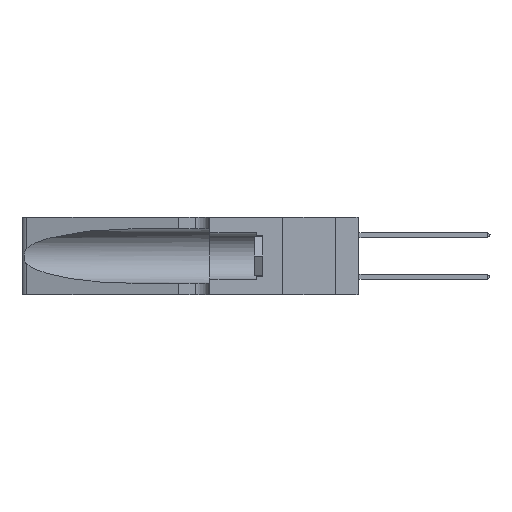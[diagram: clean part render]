
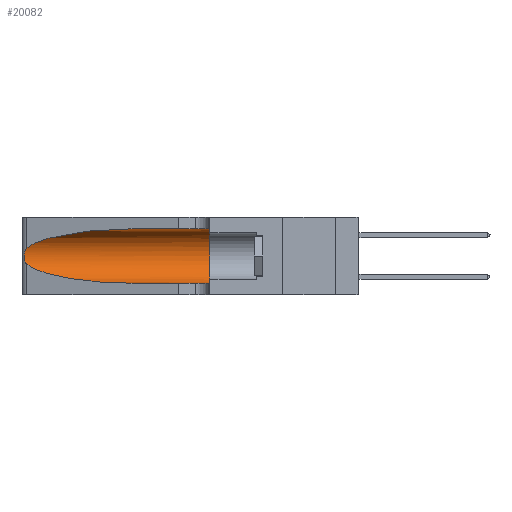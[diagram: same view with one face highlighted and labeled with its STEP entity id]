
A CAD part, left-side view. The second image highlights one B-rep face of the part: STEP entity #20082.
In plain terms, the highlighted cylindrical face has radius 3.308 mm (diameter 6.617 mm), a partial arc.
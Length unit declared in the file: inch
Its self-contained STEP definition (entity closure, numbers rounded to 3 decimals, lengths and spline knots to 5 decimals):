
#1 = VECTOR ( 'NONE', #4789, 39.37008 ) ;
#496 = VERTEX_POINT ( 'NONE', #16789 ) ;
#528 = ORIENTED_EDGE ( 'NONE', *, *, #17644, .T. ) ;
#596 = CARTESIAN_POINT ( 'NONE',  ( 0.26017, 1.23833, 0.17102 ) ) ;
#1968 = VECTOR ( 'NONE', #13540, 39.37008 ) ;
#2233 = VERTEX_POINT ( 'NONE', #7448 ) ;
#2292 = CARTESIAN_POINT ( 'NONE',  ( 0.1305, 1.61858, 0.31525 ) ) ;
#2737 = LINE ( 'NONE', #11096, #1968 ) ;
#2956 = CARTESIAN_POINT ( 'NONE',  ( 0.25555, 1.22994, 0.2215 ) ) ;
#3065 = CARTESIAN_POINT ( 'NONE',  ( 0.25789, 1.23486, 0.15765 ) ) ;
#3629 = EDGE_CURVE ( 'NONE', #496, #17994, #12127, .T. ) ;
#4636 = EDGE_CURVE ( 'NONE', #2233, #13091, #5561, .T. ) ;
#4789 = DIRECTION ( 'NONE',  ( 0., -1., 0. ) ) ;
#5550 = CARTESIAN_POINT ( 'NONE',  ( 0.25555, 1.22993, 0.14849 ) ) ;
#5561 = CIRCLE ( 'NONE', #5990, 0.13025 ) ;
#5990 = AXIS2_PLACEMENT_3D ( 'NONE', #22006, #7514, #24447 ) ;
#6458 =( BOUNDED_CURVE ( )  B_SPLINE_CURVE ( 3, ( #21441, #11854, #28164, #13734 ),
 .UNSPECIFIED., .F., .F. ) 
 B_SPLINE_CURVE_WITH_KNOTS ( ( 4, 4 ),
 ( 3.44316, 4.71239 ),
 .UNSPECIFIED. ) 
 CURVE ( )  GEOMETRIC_REPRESENTATION_ITEM ( )  RATIONAL_B_SPLINE_CURVE ( ( 1., 0.87, 0.87, 1. ) ) 
 REPRESENTATION_ITEM ( '' )  );
#7448 = CARTESIAN_POINT ( 'NONE',  ( 0.1305, 0.35, 0.31525 ) ) ;
#7514 = DIRECTION ( 'NONE',  ( 0., 1., 0. ) ) ;
#8742 = EDGE_CURVE ( 'NONE', #17994, #12324, #6458, .T. ) ;
#9635 = CARTESIAN_POINT ( 'NONE',  ( 0.2373, 1.15595, 0.28018 ) ) ;
#10351 = CARTESIAN_POINT ( 'NONE',  ( 0.25787, 1.23484, 0.2124 ) ) ;
#10816 = CARTESIAN_POINT ( 'NONE',  ( 0.25487, 1.22718, 0.14631 ) ) ;
#11096 = CARTESIAN_POINT ( 'NONE',  ( 0.1305, 1.61858, 0.05475 ) ) ;
#11854 = CARTESIAN_POINT ( 'NONE',  ( 0.2373, 1.15595, 0.08982 ) ) ;
#11987 = CARTESIAN_POINT ( 'NONE',  ( 0.18966, 0.96281, 0.31525 ) ) ;
#12127 = B_SPLINE_CURVE_WITH_KNOTS ( 'NONE', 3,
 ( #29557, #2956, #24833, #10351, #27231, #12792, #29659, #15218, #596, #17648, #3065, #20070, #5550, #22483 ),
 .UNSPECIFIED., .F., .F.,
 ( 4, 2, 2, 2, 2, 2, 4 ),
 ( 0., 0.00027, 0.00053, 0.00107, 0.0016, 0.00187, 0.00214 ),
 .UNSPECIFIED. ) ;
#12265 = VERTEX_POINT ( 'NONE', #16935 ) ;
#12316 = CARTESIAN_POINT ( 'NONE',  ( 0.1305, 0.72297, 0.05475 ) ) ;
#12324 = VERTEX_POINT ( 'NONE', #12316 ) ;
#12792 = CARTESIAN_POINT ( 'NONE',  ( 0.26018, 1.23835, 0.19895 ) ) ;
#13091 = VERTEX_POINT ( 'NONE', #19764 ) ;
#13110 = CYLINDRICAL_SURFACE ( 'NONE', #20943, 0.13025 ) ;
#13540 = DIRECTION ( 'NONE',  ( 0., -1., 0. ) ) ;
#13734 = CARTESIAN_POINT ( 'NONE',  ( 0.1305, 0.72297, 0.05475 ) ) ;
#14319 = CARTESIAN_POINT ( 'NONE',  ( 0.1305, 0.72297, 0.31525 ) ) ;
#14555 = DIRECTION ( 'NONE',  ( 0., 0., -1. ) ) ;
#14659 = ORIENTED_EDGE ( 'NONE', *, *, #3629, .T. ) ;
#15218 = CARTESIAN_POINT ( 'NONE',  ( 0.26075, 1.23896, 0.178 ) ) ;
#15238 = EDGE_LOOP ( 'NONE', ( #528, #14659, #27485, #29419, #21823, #20385 ) ) ;
#16789 = CARTESIAN_POINT ( 'NONE',  ( 0.25487, 1.22718, 0.22369 ) ) ;
#16935 = CARTESIAN_POINT ( 'NONE',  ( 0.1305, 0.72297, 0.31525 ) ) ;
#16963 = DIRECTION ( 'NONE',  ( 0., -1., 0. ) ) ;
#17644 = EDGE_CURVE ( 'NONE', #12265, #496, #21013, .T. ) ;
#17648 = CARTESIAN_POINT ( 'NONE',  ( 0.25856, 1.23593, 0.16098 ) ) ;
#17994 = VERTEX_POINT ( 'NONE', #10816 ) ;
#19459 = LINE ( 'NONE', #2292, #1 ) ;
#19764 = CARTESIAN_POINT ( 'NONE',  ( 0.1305, 0.35, 0.05475 ) ) ;
#20070 = CARTESIAN_POINT ( 'NONE',  ( 0.25639, 1.23186, 0.15144 ) ) ;
#20082 = ADVANCED_FACE ( 'NONE', ( #26675 ), #13110, .F. ) ;
#20385 = ORIENTED_EDGE ( 'NONE', *, *, #20900, .F. ) ;
#20900 = EDGE_CURVE ( 'NONE', #12265, #2233, #19459, .T. ) ;
#20943 = AXIS2_PLACEMENT_3D ( 'NONE', #31371, #16963, #14555 ) ;
#21013 =( BOUNDED_CURVE ( )  B_SPLINE_CURVE ( 3, ( #14319, #11987, #9635, #26526 ),
 .UNSPECIFIED., .F., .F. ) 
 B_SPLINE_CURVE_WITH_KNOTS ( ( 4, 4 ),
 ( 1.5708, 2.84003 ),
 .UNSPECIFIED. ) 
 CURVE ( )  GEOMETRIC_REPRESENTATION_ITEM ( )  RATIONAL_B_SPLINE_CURVE ( ( 1., 0.87, 0.87, 1. ) ) 
 REPRESENTATION_ITEM ( '' )  );
#21441 = CARTESIAN_POINT ( 'NONE',  ( 0.25487, 1.22718, 0.14631 ) ) ;
#21823 = ORIENTED_EDGE ( 'NONE', *, *, #4636, .F. ) ;
#22006 = CARTESIAN_POINT ( 'NONE',  ( 0.1305, 0.35, 0.185 ) ) ;
#22483 = CARTESIAN_POINT ( 'NONE',  ( 0.25487, 1.22718, 0.14631 ) ) ;
#24447 = DIRECTION ( 'NONE',  ( 0., 0., 1. ) ) ;
#24833 = CARTESIAN_POINT ( 'NONE',  ( 0.25639, 1.23184, 0.21858 ) ) ;
#26526 = CARTESIAN_POINT ( 'NONE',  ( 0.25487, 1.22718, 0.22369 ) ) ;
#26675 = FACE_OUTER_BOUND ( 'NONE', #15238, .T. ) ;
#27231 = CARTESIAN_POINT ( 'NONE',  ( 0.25854, 1.2359, 0.20912 ) ) ;
#27485 = ORIENTED_EDGE ( 'NONE', *, *, #8742, .T. ) ;
#28164 = CARTESIAN_POINT ( 'NONE',  ( 0.18966, 0.96281, 0.05475 ) ) ;
#29419 = ORIENTED_EDGE ( 'NONE', *, *, #29594, .T. ) ;
#29557 = CARTESIAN_POINT ( 'NONE',  ( 0.25487, 1.22718, 0.22369 ) ) ;
#29594 = EDGE_CURVE ( 'NONE', #12324, #13091, #2737, .T. ) ;
#29659 = CARTESIAN_POINT ( 'NONE',  ( 0.26075, 1.23896, 0.19203 ) ) ;
#31371 = CARTESIAN_POINT ( 'NONE',  ( 0.1305, 1.61858, 0.185 ) ) ;
